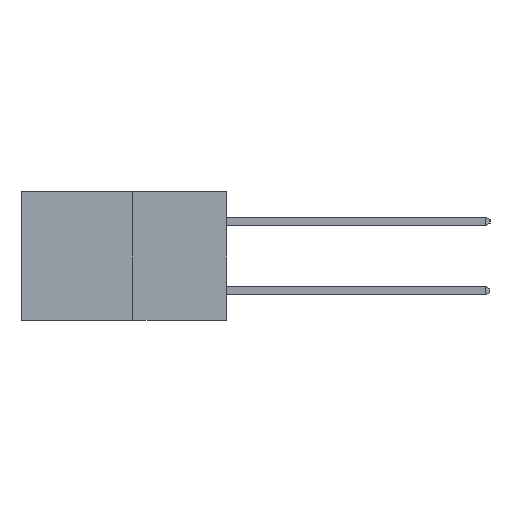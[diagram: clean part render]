
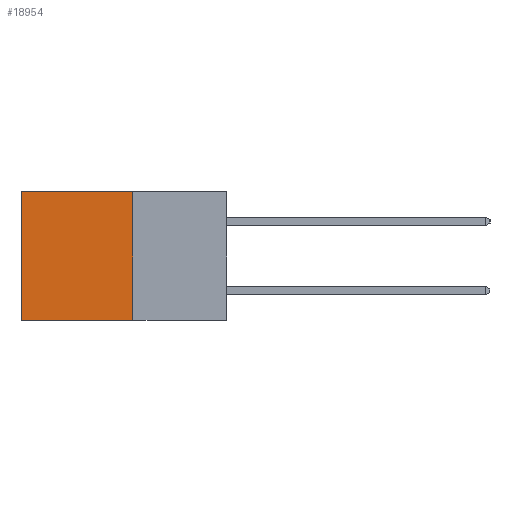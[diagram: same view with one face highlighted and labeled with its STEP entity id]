
A CAD part, left-side view. The second image highlights one B-rep face of the part: STEP entity #18954.
In plain terms, the highlighted planar face has unit normal (-1, 0, 0).
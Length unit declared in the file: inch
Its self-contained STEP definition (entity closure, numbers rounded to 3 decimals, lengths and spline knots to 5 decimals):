
#247 = CARTESIAN_POINT ( 'NONE',  ( 0.277, 0.27, 0. ) ) ;
#493 = ORIENTED_EDGE ( 'NONE', *, *, #7763, .F. ) ;
#1489 = DIRECTION ( 'NONE',  ( 0., 0., -1. ) ) ;
#1666 = EDGE_LOOP ( 'NONE', ( #8941, #6919, #493, #18397 ) ) ;
#1901 = LINE ( 'NONE', #247, #11004 ) ;
#2093 = DIRECTION ( 'NONE',  ( 0., 1., 0. ) ) ;
#2620 = CARTESIAN_POINT ( 'NONE',  ( 0.277, 0.59, 0. ) ) ;
#3222 = DIRECTION ( 'NONE',  ( 0., 0., -1. ) ) ;
#4713 = VECTOR ( 'NONE', #3222, 39.37008 ) ;
#5376 = LINE ( 'NONE', #6915, #18985 ) ;
#5538 = VERTEX_POINT ( 'NONE', #2620 ) ;
#6915 = CARTESIAN_POINT ( 'NONE',  ( 0.277, 0.27, -0.37 ) ) ;
#6919 = ORIENTED_EDGE ( 'NONE', *, *, #20875, .F. ) ;
#6987 = CARTESIAN_POINT ( 'NONE',  ( 0.277, 0.27, -0.37 ) ) ;
#7195 = VERTEX_POINT ( 'NONE', #21360 ) ;
#7763 = EDGE_CURVE ( 'NONE', #11207, #7195, #5376, .T. ) ;
#8173 = CARTESIAN_POINT ( 'NONE',  ( 0.277, 0.59, -0.37 ) ) ;
#8795 = DIRECTION ( 'NONE',  ( 0., 1., 0. ) ) ;
#8941 = ORIENTED_EDGE ( 'NONE', *, *, #20186, .T. ) ;
#9303 = AXIS2_PLACEMENT_3D ( 'NONE', #22716, #12350, #1489 ) ;
#9392 = LINE ( 'NONE', #6987, #18236 ) ;
#10577 = PLANE ( 'NONE',  #9303 ) ;
#11004 = VECTOR ( 'NONE', #2093, 39.37008 ) ;
#11207 = VERTEX_POINT ( 'NONE', #19095 ) ;
#12350 = DIRECTION ( 'NONE',  ( 1., 0., 0. ) ) ;
#15379 = VERTEX_POINT ( 'NONE', #8173 ) ;
#15853 = DIRECTION ( 'NONE',  ( 0., 0., -1. ) ) ;
#16480 = FACE_OUTER_BOUND ( 'NONE', #1666, .T. ) ;
#18236 = VECTOR ( 'NONE', #8795, 39.37008 ) ;
#18397 = ORIENTED_EDGE ( 'NONE', *, *, #22708, .T. ) ;
#18954 = ADVANCED_FACE ( 'NONE', ( #16480 ), #10577, .F. ) ;
#18985 = VECTOR ( 'NONE', #15853, 39.37008 ) ;
#19095 = CARTESIAN_POINT ( 'NONE',  ( 0.277, 0.27, 0. ) ) ;
#19289 = CARTESIAN_POINT ( 'NONE',  ( 0.277, 0.59, -0.37 ) ) ;
#20186 = EDGE_CURVE ( 'NONE', #5538, #15379, #22843, .T. ) ;
#20875 = EDGE_CURVE ( 'NONE', #7195, #15379, #9392, .T. ) ;
#21360 = CARTESIAN_POINT ( 'NONE',  ( 0.277, 0.27, -0.37 ) ) ;
#22708 = EDGE_CURVE ( 'NONE', #11207, #5538, #1901, .T. ) ;
#22716 = CARTESIAN_POINT ( 'NONE',  ( 0.277, 0.27, -0.37 ) ) ;
#22843 = LINE ( 'NONE', #19289, #4713 ) ;
